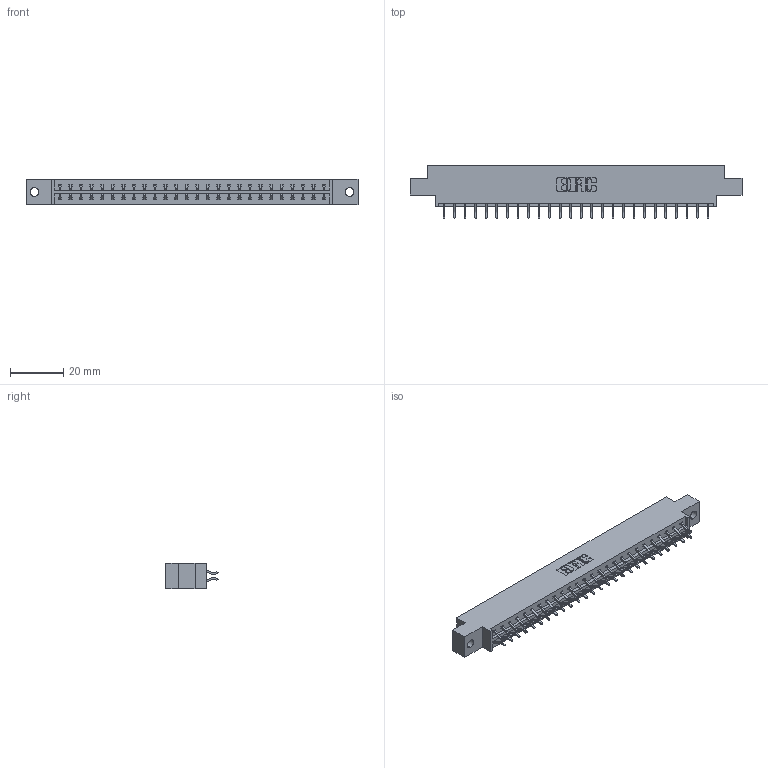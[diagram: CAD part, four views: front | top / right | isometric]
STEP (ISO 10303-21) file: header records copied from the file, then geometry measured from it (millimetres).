
FILE_DESCRIPTION (( 'STEP AP203' ), '1' );
FILE_NAME ('333-052-556-802.STEP', '2018-08-04T03:09:42', ( '' ), ( '' ), 'SwSTEP 2.0', 'SolidWorks 2016', '' );
FILE_SCHEMA (( 'CONFIG_CONTROL_DESIGN' ));
Length unit declared in the file: inch
Products named in the file (3): 333 Part_Offset - .128 Dia; 345-292-001_556 Tail; 333-052-556-802
Assembly tree (53 placements, depth 2):
  333-052-556-802
    333 Part_Offset - .128 Dia
    345-292-001_556 Tail  x52
Bounding box: 124.56 x 19.57 x 9.4 mm (x, y, z)
Volume: 12300.9 mm3; surface area: 14267 mm2
Topology: 53 solids, 53 shells, 3134 faces, 9319 edges, 6142 vertices
Faces by surface type: plane 2154, cylinder 980
Entity records: 19151 total; most frequent: CARTESIAN_POINT 3210, ORIENTED_EDGE 3134, DIRECTION 2759, EDGE_CURVE 1567, LINE 1431, VECTOR 1431, VERTEX_POINT 1042, AXIS2_PLACEMENT_3D 664
